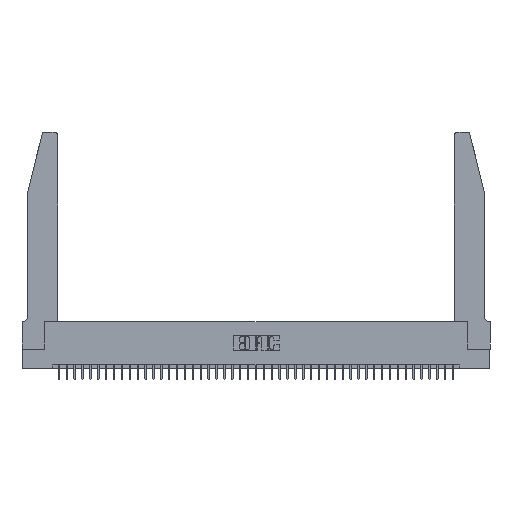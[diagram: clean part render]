
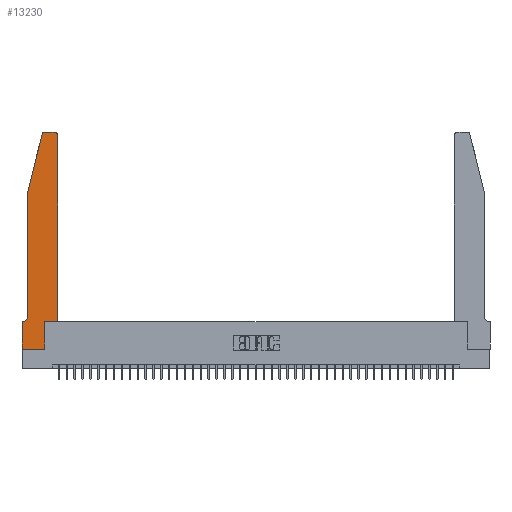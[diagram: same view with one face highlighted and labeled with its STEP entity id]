
A CAD part, top view. The second image highlights one B-rep face of the part: STEP entity #13230.
In plain terms, the highlighted planar face has unit normal (0, 0, 1).
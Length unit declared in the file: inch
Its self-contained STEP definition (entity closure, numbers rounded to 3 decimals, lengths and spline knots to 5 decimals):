
#224 = CARTESIAN_POINT ( 'NONE',  ( 0.284, 2.72, 0.37 ) ) ;
#611 = DIRECTION ( 'NONE',  ( 1., 0., 0. ) ) ;
#1033 = VECTOR ( 'NONE', #22548, 39.37008 ) ;
#1584 = EDGE_CURVE ( 'NONE', #40161, #34313, #32518, .T. ) ;
#1655 = VECTOR ( 'NONE', #17572, 39.37008 ) ;
#2817 = CARTESIAN_POINT ( 'NONE',  ( 0., 0.35, 0.37 ) ) ;
#4102 = CARTESIAN_POINT ( 'NONE',  ( 0.0755, 2., 0.37 ) ) ;
#4649 = ORIENTED_EDGE ( 'NONE', *, *, #33225, .T. ) ;
#4653 = VERTEX_POINT ( 'NONE', #24109 ) ;
#4883 = EDGE_CURVE ( 'NONE', #38601, #40161, #42648, .T. ) ;
#4893 = DIRECTION ( 'NONE',  ( 0., -1., 0. ) ) ;
#5117 = VECTOR ( 'NONE', #32918, 39.37008 ) ;
#7135 = DIRECTION ( 'NONE',  ( 0., -1., 0. ) ) ;
#7293 = LINE ( 'NONE', #37784, #34554 ) ;
#7507 = DIRECTION ( 'NONE',  ( 0., 1., 0. ) ) ;
#7624 = VERTEX_POINT ( 'NONE', #27424 ) ;
#7742 = DIRECTION ( 'NONE',  ( 0., 0., -1. ) ) ;
#8396 = LINE ( 'NONE', #18766, #5117 ) ;
#8832 = CARTESIAN_POINT ( 'NONE',  ( 0.2865, 0.35, 0.37 ) ) ;
#9032 = CARTESIAN_POINT ( 'NONE',  ( 0.4205, 2.72, 0.37 ) ) ;
#9513 = ORIENTED_EDGE ( 'NONE', *, *, #1584, .T. ) ;
#10247 = CIRCLE ( 'NONE', #20167, 0.07 ) ;
#10594 = DIRECTION ( 'NONE',  ( 0., 0., 1. ) ) ;
#10642 = LINE ( 'NONE', #24145, #11499 ) ;
#10656 = LINE ( 'NONE', #30765, #28251 ) ;
#11269 = DIRECTION ( 'NONE',  ( -1., 0., 0. ) ) ;
#11288 = VERTEX_POINT ( 'NONE', #37126 ) ;
#11455 = CARTESIAN_POINT ( 'NONE',  ( 0.4505, 0.35, 0.37 ) ) ;
#11499 = VECTOR ( 'NONE', #20793, 39.37008 ) ;
#11697 = DIRECTION ( 'NONE',  ( 1., 0., 0. ) ) ;
#12273 = EDGE_CURVE ( 'NONE', #34313, #18056, #34209, .T. ) ;
#12531 = ORIENTED_EDGE ( 'NONE', *, *, #12273, .T. ) ;
#13230 = ADVANCED_FACE ( 'NONE', ( #21228 ), #21442, .T. ) ;
#13361 = VERTEX_POINT ( 'NONE', #32500 ) ;
#13419 = EDGE_CURVE ( 'NONE', #38319, #28552, #8396, .T. ) ;
#16297 = DIRECTION ( 'NONE',  ( 1., 0., 0. ) ) ;
#16390 = AXIS2_PLACEMENT_3D ( 'NONE', #41795, #25001, #18115 ) ;
#16490 = ORIENTED_EDGE ( 'NONE', *, *, #42099, .T. ) ;
#17178 = ORIENTED_EDGE ( 'NONE', *, *, #42522, .T. ) ;
#17207 = ORIENTED_EDGE ( 'NONE', *, *, #28384, .T. ) ;
#17572 = DIRECTION ( 'NONE',  ( -0.239, -0.971, 0. ) ) ;
#17775 = ORIENTED_EDGE ( 'NONE', *, *, #38343, .T. ) ;
#18056 = VERTEX_POINT ( 'NONE', #11455 ) ;
#18115 = DIRECTION ( 'NONE',  ( 1., 0., 0. ) ) ;
#18421 = VERTEX_POINT ( 'NONE', #23801 ) ;
#18766 = CARTESIAN_POINT ( 'NONE',  ( 0.0755, 0.35, 0.37 ) ) ;
#19630 = VERTEX_POINT ( 'NONE', #28227 ) ;
#19652 = CARTESIAN_POINT ( 'NONE',  ( 0.2865, 0.35, 0.37 ) ) ;
#20167 = AXIS2_PLACEMENT_3D ( 'NONE', #35147, #7742, #11269 ) ;
#20793 = DIRECTION ( 'NONE',  ( -1., 0., 0. ) ) ;
#20901 = LINE ( 'NONE', #4102, #1655 ) ;
#21228 = FACE_OUTER_BOUND ( 'NONE', #41590, .T. ) ;
#21311 = CIRCLE ( 'NONE', #22012, 0.03 ) ;
#21341 = AXIS2_PLACEMENT_3D ( 'NONE', #224, #10594, #24102 ) ;
#21442 = PLANE ( 'NONE',  #16390 ) ;
#22012 = AXIS2_PLACEMENT_3D ( 'NONE', #9032, #25425, #11697 ) ;
#22548 = DIRECTION ( 'NONE',  ( 0., 1., 0. ) ) ;
#23039 = ORIENTED_EDGE ( 'NONE', *, *, #43205, .T. ) ;
#23801 = CARTESIAN_POINT ( 'NONE',  ( 0.4505, 2.72, 0.37 ) ) ;
#24102 = DIRECTION ( 'NONE',  ( 1., 0., 0. ) ) ;
#24109 = CARTESIAN_POINT ( 'NONE',  ( 0.0755, 0.42, 0.37 ) ) ;
#24145 = CARTESIAN_POINT ( 'NONE',  ( 0.2605, 2.75, 0.37 ) ) ;
#24543 = CARTESIAN_POINT ( 'NONE',  ( 0.0055, 0.35, 0.37 ) ) ;
#25001 = DIRECTION ( 'NONE',  ( 0., 0., 1. ) ) ;
#25425 = DIRECTION ( 'NONE',  ( 0., 0., 1. ) ) ;
#26229 = CARTESIAN_POINT ( 'NONE',  ( 0.2865, 0., 0.37 ) ) ;
#26853 = EDGE_CURVE ( 'NONE', #18421, #13361, #21311, .T. ) ;
#27137 = ORIENTED_EDGE ( 'NONE', *, *, #13419, .T. ) ;
#27424 = CARTESIAN_POINT ( 'NONE',  ( 0.284, 2.75, 0.37 ) ) ;
#28227 = CARTESIAN_POINT ( 'NONE',  ( 0.25487, 2.72718, 0.37 ) ) ;
#28251 = VECTOR ( 'NONE', #7135, 39.37008 ) ;
#28384 = EDGE_CURVE ( 'NONE', #13361, #7624, #10642, .T. ) ;
#28552 = VERTEX_POINT ( 'NONE', #2817 ) ;
#30011 = EDGE_CURVE ( 'NONE', #7624, #19630, #32644, .T. ) ;
#30667 = CARTESIAN_POINT ( 'NONE',  ( 0.4505, 0.35, 0.37 ) ) ;
#30765 = CARTESIAN_POINT ( 'NONE',  ( 0.0755, 2., 0.37 ) ) ;
#31161 = VECTOR ( 'NONE', #611, 39.37008 ) ;
#32500 = CARTESIAN_POINT ( 'NONE',  ( 0.4205, 2.75, 0.37 ) ) ;
#32518 = LINE ( 'NONE', #8832, #1033 ) ;
#32631 = ORIENTED_EDGE ( 'NONE', *, *, #4883, .T. ) ;
#32644 = CIRCLE ( 'NONE', #21341, 0.03 ) ;
#32898 = CARTESIAN_POINT ( 'NONE',  ( 0., 0., 0.37 ) ) ;
#32918 = DIRECTION ( 'NONE',  ( -1., 0., 0. ) ) ;
#33225 = EDGE_CURVE ( 'NONE', #19630, #11288, #20901, .T. ) ;
#33679 = VECTOR ( 'NONE', #16297, 39.37008 ) ;
#34209 = LINE ( 'NONE', #30667, #31161 ) ;
#34313 = VERTEX_POINT ( 'NONE', #19652 ) ;
#34554 = VECTOR ( 'NONE', #7507, 39.37008 ) ;
#35147 = CARTESIAN_POINT ( 'NONE',  ( 0.0055, 0.42, 0.37 ) ) ;
#35187 = CARTESIAN_POINT ( 'NONE',  ( 0., 0., 0.37 ) ) ;
#36458 = CARTESIAN_POINT ( 'NONE',  ( 0., 0., 0.37 ) ) ;
#37126 = CARTESIAN_POINT ( 'NONE',  ( 0.0755, 2., 0.37 ) ) ;
#37784 = CARTESIAN_POINT ( 'NONE',  ( 0.4505, 0.35, 0.37 ) ) ;
#38319 = VERTEX_POINT ( 'NONE', #24543 ) ;
#38343 = EDGE_CURVE ( 'NONE', #4653, #38319, #10247, .T. ) ;
#38601 = VERTEX_POINT ( 'NONE', #36458 ) ;
#40161 = VERTEX_POINT ( 'NONE', #26229 ) ;
#40861 = ORIENTED_EDGE ( 'NONE', *, *, #30011, .T. ) ;
#41590 = EDGE_LOOP ( 'NONE', ( #17207, #40861, #4649, #23039, #17775, #27137, #16490, #32631, #9513, #12531, #17178, #41875 ) ) ;
#41795 = CARTESIAN_POINT ( 'NONE',  ( 0., 0.35, 0.37 ) ) ;
#41825 = LINE ( 'NONE', #35187, #42290 ) ;
#41875 = ORIENTED_EDGE ( 'NONE', *, *, #26853, .T. ) ;
#42099 = EDGE_CURVE ( 'NONE', #28552, #38601, #41825, .T. ) ;
#42290 = VECTOR ( 'NONE', #4893, 39.37008 ) ;
#42522 = EDGE_CURVE ( 'NONE', #18056, #18421, #7293, .T. ) ;
#42648 = LINE ( 'NONE', #32898, #33679 ) ;
#43205 = EDGE_CURVE ( 'NONE', #11288, #4653, #10656, .T. ) ;
